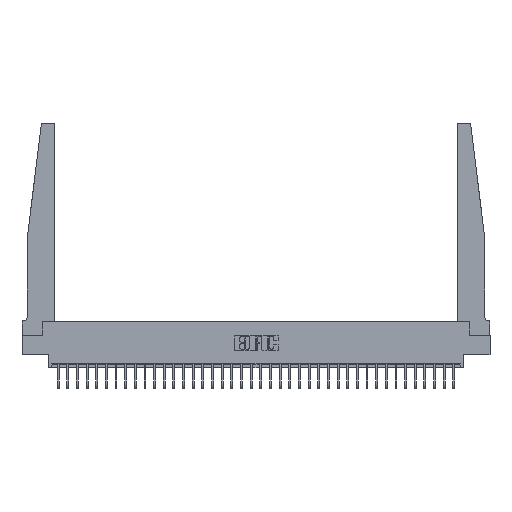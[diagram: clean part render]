
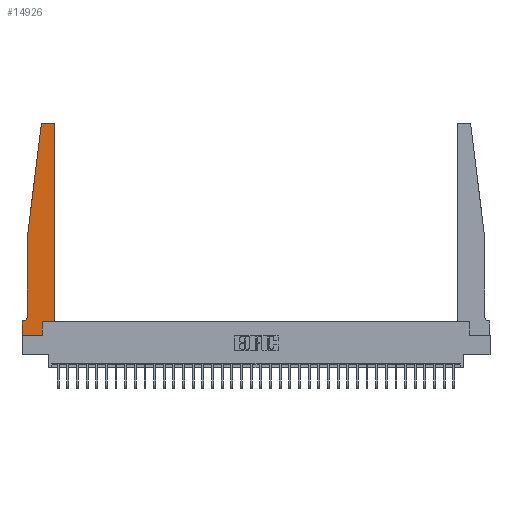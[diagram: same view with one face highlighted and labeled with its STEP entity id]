
A CAD part, top view. The second image highlights one B-rep face of the part: STEP entity #14926.
In plain terms, the highlighted planar face has unit normal (0, 0, 1).
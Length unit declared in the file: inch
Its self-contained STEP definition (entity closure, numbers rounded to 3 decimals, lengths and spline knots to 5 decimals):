
#189 = LINE ( 'NONE', #14378, #23868 ) ;
#1048 = ORIENTED_EDGE ( 'NONE', *, *, #22334, .T. ) ;
#1254 = DIRECTION ( 'NONE',  ( 1., 0., 0. ) ) ;
#1406 = CARTESIAN_POINT ( 'NONE',  ( 0.395, 2.75, 0.37 ) ) ;
#1567 = CARTESIAN_POINT ( 'NONE',  ( 0.425, 0.18, 0.37 ) ) ;
#1622 = VERTEX_POINT ( 'NONE', #17671 ) ;
#1716 = EDGE_CURVE ( 'NONE', #19545, #29470, #6180, .T. ) ;
#2338 = DIRECTION ( 'NONE',  ( 0., 1., 0. ) ) ;
#2827 = CARTESIAN_POINT ( 'NONE',  ( 0.065, 0.2375, 0.37 ) ) ;
#3192 = EDGE_CURVE ( 'NONE', #5822, #13815, #23653, .T. ) ;
#3594 = EDGE_CURVE ( 'NONE', #11561, #5822, #30514, .T. ) ;
#4302 = ORIENTED_EDGE ( 'NONE', *, *, #20974, .T. ) ;
#5024 = VECTOR ( 'NONE', #12753, 39.37008 ) ;
#5079 = VERTEX_POINT ( 'NONE', #17228 ) ;
#5234 = DIRECTION ( 'NONE',  ( 0., -1., 0. ) ) ;
#5546 = VECTOR ( 'NONE', #18403, 39.37008 ) ;
#5585 = VERTEX_POINT ( 'NONE', #8245 ) ;
#5605 = CARTESIAN_POINT ( 'NONE',  ( 0., 0., 0.37 ) ) ;
#5822 = VERTEX_POINT ( 'NONE', #1406 ) ;
#6107 = VECTOR ( 'NONE', #24894, 39.37008 ) ;
#6112 = DIRECTION ( 'NONE',  ( 0., 0., -1. ) ) ;
#6180 = LINE ( 'NONE', #1567, #11686 ) ;
#6289 = ORIENTED_EDGE ( 'NONE', *, *, #1716, .T. ) ;
#6858 = AXIS2_PLACEMENT_3D ( 'NONE', #14195, #28846, #26143 ) ;
#7586 = VECTOR ( 'NONE', #5234, 39.37008 ) ;
#7968 = CARTESIAN_POINT ( 'NONE',  ( 0.065, 1.25, 0.37 ) ) ;
#8121 = AXIS2_PLACEMENT_3D ( 'NONE', #30937, #25530, #16122 ) ;
#8245 = CARTESIAN_POINT ( 'NONE',  ( 0., 0.1875, 0.37 ) ) ;
#8888 = EDGE_CURVE ( 'NONE', #1622, #5079, #23558, .T. ) ;
#10145 = DIRECTION ( 'NONE',  ( 0., 0., 1. ) ) ;
#10525 = EDGE_CURVE ( 'NONE', #11431, #14358, #18612, .T. ) ;
#10839 = VERTEX_POINT ( 'NONE', #20746 ) ;
#11207 = CARTESIAN_POINT ( 'NONE',  ( 0.015, 0.1875, 0.37 ) ) ;
#11418 = EDGE_CURVE ( 'NONE', #13815, #1622, #16458, .T. ) ;
#11431 = VERTEX_POINT ( 'NONE', #2827 ) ;
#11561 = VERTEX_POINT ( 'NONE', #13333 ) ;
#11686 = VECTOR ( 'NONE', #1254, 39.37008 ) ;
#11799 = FACE_OUTER_BOUND ( 'NONE', #29388, .T. ) ;
#11832 = VERTEX_POINT ( 'NONE', #26981 ) ;
#12232 = CARTESIAN_POINT ( 'NONE',  ( 0.27653, 2.72, 0.37 ) ) ;
#12255 = VECTOR ( 'NONE', #12511, 39.37008 ) ;
#12276 = CARTESIAN_POINT ( 'NONE',  ( 0.425, 0.18, 0.37 ) ) ;
#12511 = DIRECTION ( 'NONE',  ( 0., 1., 0. ) ) ;
#12602 = LINE ( 'NONE', #7968, #5024 ) ;
#12753 = DIRECTION ( 'NONE',  ( 0., -1., 0. ) ) ;
#13137 = CARTESIAN_POINT ( 'NONE',  ( 0.015, 0.2375, 0.37 ) ) ;
#13333 = CARTESIAN_POINT ( 'NONE',  ( 0.425, 2.72, 0.37 ) ) ;
#13617 = CARTESIAN_POINT ( 'NONE',  ( 0.25, 2.75, 0.37 ) ) ;
#13815 = VERTEX_POINT ( 'NONE', #17033 ) ;
#13886 = VECTOR ( 'NONE', #20852, 39.37008 ) ;
#14195 = CARTESIAN_POINT ( 'NONE',  ( 0., 0.1875, 0.37 ) ) ;
#14358 = VERTEX_POINT ( 'NONE', #11207 ) ;
#14378 = CARTESIAN_POINT ( 'NONE',  ( 0.065, 0.1875, 0.37 ) ) ;
#14448 = CARTESIAN_POINT ( 'NONE',  ( 0.425, 0.18, 0.37 ) ) ;
#14926 = ADVANCED_FACE ( 'NONE', ( #11799 ), #23443, .T. ) ;
#14997 = VECTOR ( 'NONE', #2338, 39.37008 ) ;
#15250 = ORIENTED_EDGE ( 'NONE', *, *, #3594, .T. ) ;
#15866 = ORIENTED_EDGE ( 'NONE', *, *, #10525, .T. ) ;
#16122 = DIRECTION ( 'NONE',  ( 1., 0., 0. ) ) ;
#16458 = CIRCLE ( 'NONE', #23077, 0.03 ) ;
#16683 = LINE ( 'NONE', #14448, #14997 ) ;
#17033 = CARTESIAN_POINT ( 'NONE',  ( 0.27653, 2.75, 0.37 ) ) ;
#17228 = CARTESIAN_POINT ( 'NONE',  ( 0.065, 1.25, 0.37 ) ) ;
#17671 = CARTESIAN_POINT ( 'NONE',  ( 0.24675, 2.72367, 0.37 ) ) ;
#18403 = DIRECTION ( 'NONE',  ( -1., 0., 0. ) ) ;
#18612 = CIRCLE ( 'NONE', #21645, 0.05 ) ;
#19256 = DIRECTION ( 'NONE',  ( 1., 0., 0. ) ) ;
#19545 = VERTEX_POINT ( 'NONE', #27764 ) ;
#20532 = ORIENTED_EDGE ( 'NONE', *, *, #8888, .T. ) ;
#20746 = CARTESIAN_POINT ( 'NONE',  ( 0.2605, 0., 0.37 ) ) ;
#20852 = DIRECTION ( 'NONE',  ( -0.122, -0.992, 0. ) ) ;
#20974 = EDGE_CURVE ( 'NONE', #14358, #5585, #189, .T. ) ;
#21178 = EDGE_CURVE ( 'NONE', #5079, #11431, #12602, .T. ) ;
#21416 = ORIENTED_EDGE ( 'NONE', *, *, #23557, .T. ) ;
#21639 = EDGE_CURVE ( 'NONE', #5585, #11832, #22285, .T. ) ;
#21645 = AXIS2_PLACEMENT_3D ( 'NONE', #13137, #6112, #22858 ) ;
#21918 = LINE ( 'NONE', #25958, #12255 ) ;
#22129 = CARTESIAN_POINT ( 'NONE',  ( 0., 0., 0.37 ) ) ;
#22285 = LINE ( 'NONE', #22129, #7586 ) ;
#22334 = EDGE_CURVE ( 'NONE', #11832, #10839, #27282, .T. ) ;
#22858 = DIRECTION ( 'NONE',  ( -1., 0., 0. ) ) ;
#23077 = AXIS2_PLACEMENT_3D ( 'NONE', #12232, #10145, #19256 ) ;
#23443 = PLANE ( 'NONE',  #6858 ) ;
#23557 = EDGE_CURVE ( 'NONE', #10839, #19545, #21918, .T. ) ;
#23558 = LINE ( 'NONE', #25797, #13886 ) ;
#23653 = LINE ( 'NONE', #13617, #5546 ) ;
#23868 = VECTOR ( 'NONE', #26174, 39.37008 ) ;
#24149 = ORIENTED_EDGE ( 'NONE', *, *, #31282, .T. ) ;
#24894 = DIRECTION ( 'NONE',  ( 1., 0., 0. ) ) ;
#25420 = ORIENTED_EDGE ( 'NONE', *, *, #3192, .T. ) ;
#25530 = DIRECTION ( 'NONE',  ( 0., 0., 1. ) ) ;
#25797 = CARTESIAN_POINT ( 'NONE',  ( 0.065, 1.25, 0.37 ) ) ;
#25958 = CARTESIAN_POINT ( 'NONE',  ( 0.2605, 0.18, 0.37 ) ) ;
#26143 = DIRECTION ( 'NONE',  ( 1., 0., 0. ) ) ;
#26174 = DIRECTION ( 'NONE',  ( -1., 0., 0. ) ) ;
#26981 = CARTESIAN_POINT ( 'NONE',  ( 0., 0., 0.37 ) ) ;
#27282 = LINE ( 'NONE', #5605, #6107 ) ;
#27764 = CARTESIAN_POINT ( 'NONE',  ( 0.2605, 0.18, 0.37 ) ) ;
#28846 = DIRECTION ( 'NONE',  ( 0., 0., 1. ) ) ;
#28937 = ORIENTED_EDGE ( 'NONE', *, *, #21178, .T. ) ;
#29387 = ORIENTED_EDGE ( 'NONE', *, *, #21639, .T. ) ;
#29388 = EDGE_LOOP ( 'NONE', ( #25420, #29895, #20532, #28937, #15866, #4302, #29387, #1048, #21416, #6289, #24149, #15250 ) ) ;
#29470 = VERTEX_POINT ( 'NONE', #12276 ) ;
#29895 = ORIENTED_EDGE ( 'NONE', *, *, #11418, .T. ) ;
#30514 = CIRCLE ( 'NONE', #8121, 0.03 ) ;
#30937 = CARTESIAN_POINT ( 'NONE',  ( 0.395, 2.72, 0.37 ) ) ;
#31282 = EDGE_CURVE ( 'NONE', #29470, #11561, #16683, .T. ) ;
